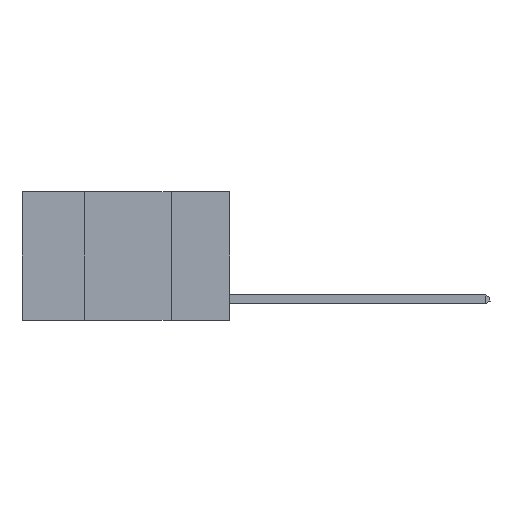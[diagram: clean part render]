
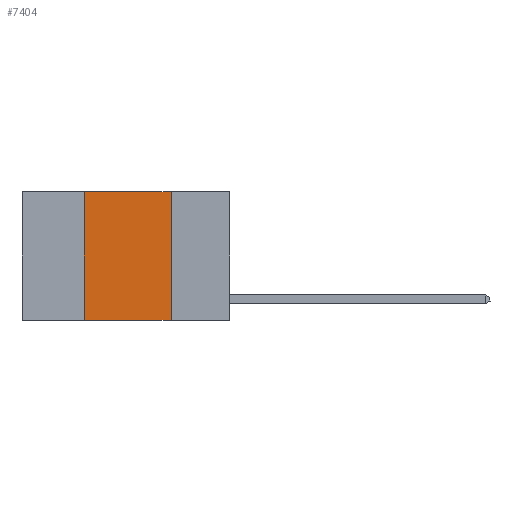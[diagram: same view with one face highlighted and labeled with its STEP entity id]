
A CAD part, left-side view. The second image highlights one B-rep face of the part: STEP entity #7404.
In plain terms, the highlighted planar face has unit normal (-1, 0, 0).
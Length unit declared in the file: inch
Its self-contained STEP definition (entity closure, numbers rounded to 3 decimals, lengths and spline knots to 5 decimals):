
#196 = ORIENTED_EDGE ( 'NONE', *, *, #2184, .F. ) ;
#355 = ORIENTED_EDGE ( 'NONE', *, *, #2494, .F. ) ;
#1394 = VECTOR ( 'NONE', #3157, 39.37008 ) ;
#1468 = FACE_OUTER_BOUND ( 'NONE', #9105, .T. ) ;
#1575 = VECTOR ( 'NONE', #8833, 39.37008 ) ;
#2169 = CARTESIAN_POINT ( 'NONE',  ( 0., 0.6, 0. ) ) ;
#2184 = EDGE_CURVE ( 'NONE', #8312, #6172, #11206, .T. ) ;
#2271 = EDGE_CURVE ( 'NONE', #4855, #8569, #7667, .T. ) ;
#2375 = VECTOR ( 'NONE', #6902, 39.37008 ) ;
#2494 = EDGE_CURVE ( 'NONE', #8569, #8312, #6817, .T. ) ;
#2573 = LINE ( 'NONE', #7292, #1575 ) ;
#2619 = CARTESIAN_POINT ( 'NONE',  ( 0., 0.42, -0.37 ) ) ;
#3157 = DIRECTION ( 'NONE',  ( 0., 0., -1. ) ) ;
#3251 = DIRECTION ( 'NONE',  ( 0., 0., -1. ) ) ;
#3972 = ORIENTED_EDGE ( 'NONE', *, *, #2271, .F. ) ;
#3987 = EDGE_CURVE ( 'NONE', #4855, #6172, #2573, .T. ) ;
#4272 = CARTESIAN_POINT ( 'NONE',  ( 0., 0.42, 0. ) ) ;
#4855 = VERTEX_POINT ( 'NONE', #2619 ) ;
#5747 = AXIS2_PLACEMENT_3D ( 'NONE', #2169, #8602, #3251 ) ;
#5907 = CARTESIAN_POINT ( 'NONE',  ( 0., 0.17, -0.37 ) ) ;
#6172 = VERTEX_POINT ( 'NONE', #5907 ) ;
#6817 = LINE ( 'NONE', #11237, #8645 ) ;
#6902 = DIRECTION ( 'NONE',  ( 0., 0., 1. ) ) ;
#7292 = CARTESIAN_POINT ( 'NONE',  ( 0., 0.6, -0.37 ) ) ;
#7404 = ADVANCED_FACE ( 'NONE', ( #1468 ), #10252, .F. ) ;
#7667 = LINE ( 'NONE', #4272, #2375 ) ;
#8052 = ORIENTED_EDGE ( 'NONE', *, *, #3987, .T. ) ;
#8247 = CARTESIAN_POINT ( 'NONE',  ( 0., 0.42, 0. ) ) ;
#8312 = VERTEX_POINT ( 'NONE', #8571 ) ;
#8569 = VERTEX_POINT ( 'NONE', #8247 ) ;
#8571 = CARTESIAN_POINT ( 'NONE',  ( 0., 0.17, 0. ) ) ;
#8602 = DIRECTION ( 'NONE',  ( 1., 0., 0. ) ) ;
#8645 = VECTOR ( 'NONE', #11174, 39.37008 ) ;
#8833 = DIRECTION ( 'NONE',  ( 0., -1., 0. ) ) ;
#9105 = EDGE_LOOP ( 'NONE', ( #196, #355, #3972, #8052 ) ) ;
#10252 = PLANE ( 'NONE',  #5747 ) ;
#10954 = CARTESIAN_POINT ( 'NONE',  ( 0., 0.17, 0. ) ) ;
#11174 = DIRECTION ( 'NONE',  ( 0., -1., 0. ) ) ;
#11206 = LINE ( 'NONE', #10954, #1394 ) ;
#11237 = CARTESIAN_POINT ( 'NONE',  ( 0., 0.6, 0. ) ) ;
